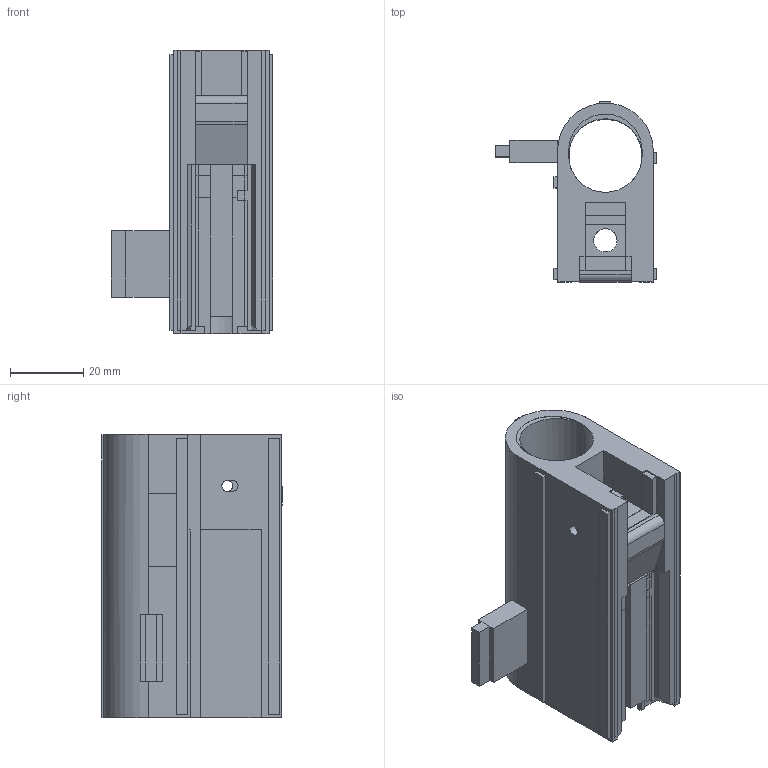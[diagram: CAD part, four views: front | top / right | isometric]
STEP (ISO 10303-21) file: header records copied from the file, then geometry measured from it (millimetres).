
FILE_DESCRIPTION (( 'STEP AP203' ), '1' );
FILE_NAME ('wtf mod9 bolt housing.STEP', '2020-08-24T00:24:54', ( '' ), ( '' ), 'SwSTEP 2.0', 'SolidWorks 2019', '' );
FILE_SCHEMA (( 'CONFIG_CONTROL_DESIGN' ));
Length unit declared in the file: millimetre
Products named in the file (1): wtf mod9 bolt housing
Bounding box: 44 x 49.1 x 77.19 mm (x, y, z)
Volume: 45382.5 mm3; surface area: 22716.6 mm2
Topology: 1 solids, 3 shells, 266 faces, 732 edges, 472 vertices
Faces by surface type: plane 242, cylinder 24
Entity records: 8621 total; most frequent: CARTESIAN_POINT 1728, ORIENTED_EDGE 1464, DIRECTION 1346, EDGE_CURVE 732, VECTOR 618, LINE 618, VERTEX_POINT 472, AXIS2_PLACEMENT_3D 364
